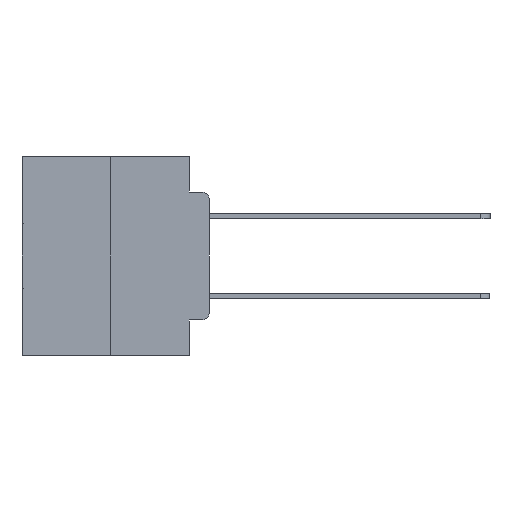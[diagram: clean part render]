
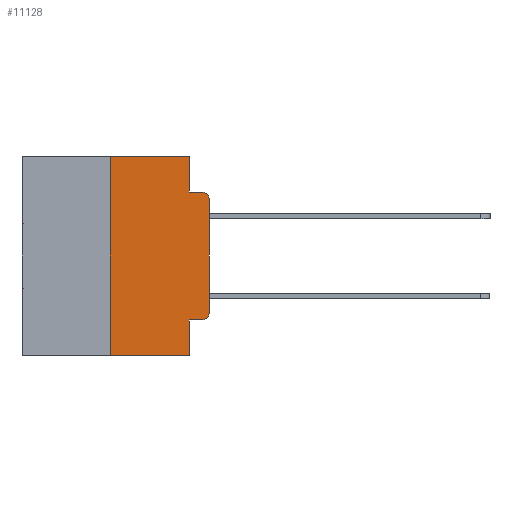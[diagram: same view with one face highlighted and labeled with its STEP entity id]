
A CAD part, left-side view. The second image highlights one B-rep face of the part: STEP entity #11128.
In plain terms, the highlighted planar face has unit normal (-1, 0, 0).
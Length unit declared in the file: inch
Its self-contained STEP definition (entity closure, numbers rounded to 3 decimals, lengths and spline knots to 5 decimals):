
#591 = VECTOR ( 'NONE', #12148, 39.37008 ) ;
#1011 = ORIENTED_EDGE ( 'NONE', *, *, #3216, .F. ) ;
#1259 = PLANE ( 'NONE',  #14337 ) ;
#1287 = VECTOR ( 'NONE', #23604, 39.37008 ) ;
#1819 = ORIENTED_EDGE ( 'NONE', *, *, #7793, .F. ) ;
#1980 = CARTESIAN_POINT ( 'NONE',  ( 0., 0.051, -0.5 ) ) ;
#2582 = CARTESIAN_POINT ( 'NONE',  ( 0., 0.02, -0.3915 ) ) ;
#2584 = ORIENTED_EDGE ( 'NONE', *, *, #12387, .T. ) ;
#3216 = EDGE_CURVE ( 'NONE', #10100, #7797, #18360, .T. ) ;
#3346 = EDGE_CURVE ( 'NONE', #12877, #4915, #8754, .T. ) ;
#3625 = DIRECTION ( 'NONE',  ( 0., -1., 0. ) ) ;
#3732 = CARTESIAN_POINT ( 'NONE',  ( 0., 0.02, -0.1085 ) ) ;
#4142 = ORIENTED_EDGE ( 'NONE', *, *, #19835, .F. ) ;
#4915 = VERTEX_POINT ( 'NONE', #19417 ) ;
#4930 = VERTEX_POINT ( 'NONE', #1980 ) ;
#4975 = DIRECTION ( 'NONE',  ( 0., 0., -1. ) ) ;
#5462 = LINE ( 'NONE', #28255, #28919 ) ;
#5467 = VERTEX_POINT ( 'NONE', #29019 ) ;
#5573 = DIRECTION ( 'NONE',  ( 0., 0., -1. ) ) ;
#5941 = EDGE_CURVE ( 'NONE', #21531, #12877, #14983, .T. ) ;
#6285 = VECTOR ( 'NONE', #28120, 39.37008 ) ;
#6635 = VECTOR ( 'NONE', #16902, 39.37008 ) ;
#7273 = EDGE_CURVE ( 'NONE', #15560, #5467, #5462, .T. ) ;
#7456 = VERTEX_POINT ( 'NONE', #19822 ) ;
#7733 = CARTESIAN_POINT ( 'NONE',  ( 0., 0.25, -0.5 ) ) ;
#7793 = EDGE_CURVE ( 'NONE', #24140, #4930, #28193, .T. ) ;
#7797 = VERTEX_POINT ( 'NONE', #21526 ) ;
#8403 = DIRECTION ( 'NONE',  ( 1., 0., 0. ) ) ;
#8754 = CIRCLE ( 'NONE', #23915, 0.02 ) ;
#8822 = DIRECTION ( 'NONE',  ( 0., -1., 0. ) ) ;
#9124 = DIRECTION ( 'NONE',  ( -1., 0., 0. ) ) ;
#9318 = VECTOR ( 'NONE', #8822, 39.37008 ) ;
#9347 = VECTOR ( 'NONE', #5573, 39.37008 ) ;
#10097 = DIRECTION ( 'NONE',  ( 0., 0., 1. ) ) ;
#10100 = VERTEX_POINT ( 'NONE', #27360 ) ;
#10915 = VECTOR ( 'NONE', #3625, 39.37008 ) ;
#11128 = ADVANCED_FACE ( 'NONE', ( #27339 ), #1259, .F. ) ;
#12137 = CARTESIAN_POINT ( 'NONE',  ( 0., 0., 0. ) ) ;
#12148 = DIRECTION ( 'NONE',  ( 0., -1., 0. ) ) ;
#12387 = EDGE_CURVE ( 'NONE', #24140, #7456, #24798, .T. ) ;
#12877 = VERTEX_POINT ( 'NONE', #18769 ) ;
#14337 = AXIS2_PLACEMENT_3D ( 'NONE', #22064, #8403, #24349 ) ;
#14983 = LINE ( 'NONE', #12137, #1287 ) ;
#15233 = EDGE_LOOP ( 'NONE', ( #20167, #18102, #19751, #1011, #4142, #17232, #20423, #1819, #2584, #26222 ) ) ;
#15560 = VERTEX_POINT ( 'NONE', #7733 ) ;
#16508 = CARTESIAN_POINT ( 'NONE',  ( 0., 0.051, -0.4115 ) ) ;
#16902 = DIRECTION ( 'NONE',  ( 0., -1., 0. ) ) ;
#17232 = ORIENTED_EDGE ( 'NONE', *, *, #7273, .F. ) ;
#17514 = EDGE_CURVE ( 'NONE', #7456, #21531, #22926, .T. ) ;
#18102 = ORIENTED_EDGE ( 'NONE', *, *, #3346, .T. ) ;
#18163 = CARTESIAN_POINT ( 'NONE',  ( 0., 0.051, 0. ) ) ;
#18360 = LINE ( 'NONE', #18163, #6285 ) ;
#18414 = CARTESIAN_POINT ( 'NONE',  ( 0., 0.051, -0.0885 ) ) ;
#18604 = DIRECTION ( 'NONE',  ( -1., 0., 0. ) ) ;
#18769 = CARTESIAN_POINT ( 'NONE',  ( 0., 0., -0.1085 ) ) ;
#19017 = CARTESIAN_POINT ( 'NONE',  ( 0., 0.473, -0.5 ) ) ;
#19417 = CARTESIAN_POINT ( 'NONE',  ( 0., 0.02, -0.0885 ) ) ;
#19751 = ORIENTED_EDGE ( 'NONE', *, *, #29530, .F. ) ;
#19822 = CARTESIAN_POINT ( 'NONE',  ( 0., 0.02, -0.4115 ) ) ;
#19835 = EDGE_CURVE ( 'NONE', #5467, #10100, #28315, .T. ) ;
#20167 = ORIENTED_EDGE ( 'NONE', *, *, #5941, .T. ) ;
#20423 = ORIENTED_EDGE ( 'NONE', *, *, #22034, .T. ) ;
#21332 = AXIS2_PLACEMENT_3D ( 'NONE', #2582, #18604, #4975 ) ;
#21451 = LINE ( 'NONE', #18414, #9318 ) ;
#21526 = CARTESIAN_POINT ( 'NONE',  ( 0., 0.051, -0.0885 ) ) ;
#21531 = VERTEX_POINT ( 'NONE', #28071 ) ;
#22034 = EDGE_CURVE ( 'NONE', #15560, #4930, #28880, .T. ) ;
#22064 = CARTESIAN_POINT ( 'NONE',  ( 0., 0.473, 0. ) ) ;
#22926 = CIRCLE ( 'NONE', #21332, 0.02 ) ;
#23604 = DIRECTION ( 'NONE',  ( 0., 0., 1. ) ) ;
#23915 = AXIS2_PLACEMENT_3D ( 'NONE', #3732, #9124, #29545 ) ;
#24140 = VERTEX_POINT ( 'NONE', #16508 ) ;
#24349 = DIRECTION ( 'NONE',  ( 0., 0., -1. ) ) ;
#24688 = CARTESIAN_POINT ( 'NONE',  ( 0., 0.473, 0. ) ) ;
#24798 = LINE ( 'NONE', #28233, #6635 ) ;
#25989 = CARTESIAN_POINT ( 'NONE',  ( 0., 0.051, 0. ) ) ;
#26222 = ORIENTED_EDGE ( 'NONE', *, *, #17514, .T. ) ;
#27339 = FACE_OUTER_BOUND ( 'NONE', #15233, .T. ) ;
#27360 = CARTESIAN_POINT ( 'NONE',  ( 0., 0.051, 0. ) ) ;
#28071 = CARTESIAN_POINT ( 'NONE',  ( 0., 0., -0.3915 ) ) ;
#28120 = DIRECTION ( 'NONE',  ( 0., 0., -1. ) ) ;
#28193 = LINE ( 'NONE', #25989, #9347 ) ;
#28233 = CARTESIAN_POINT ( 'NONE',  ( 0., 0.051, -0.4115 ) ) ;
#28255 = CARTESIAN_POINT ( 'NONE',  ( 0., 0.25, 0. ) ) ;
#28315 = LINE ( 'NONE', #24688, #10915 ) ;
#28880 = LINE ( 'NONE', #19017, #591 ) ;
#28919 = VECTOR ( 'NONE', #10097, 39.37008 ) ;
#29019 = CARTESIAN_POINT ( 'NONE',  ( 0., 0.25, 0. ) ) ;
#29530 = EDGE_CURVE ( 'NONE', #7797, #4915, #21451, .T. ) ;
#29545 = DIRECTION ( 'NONE',  ( 0., 0., -1. ) ) ;
